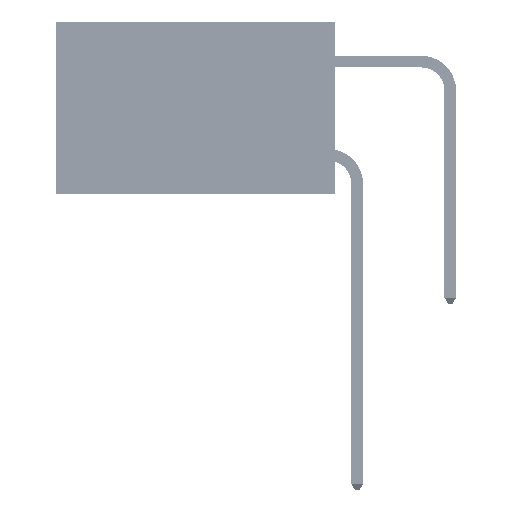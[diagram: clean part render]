
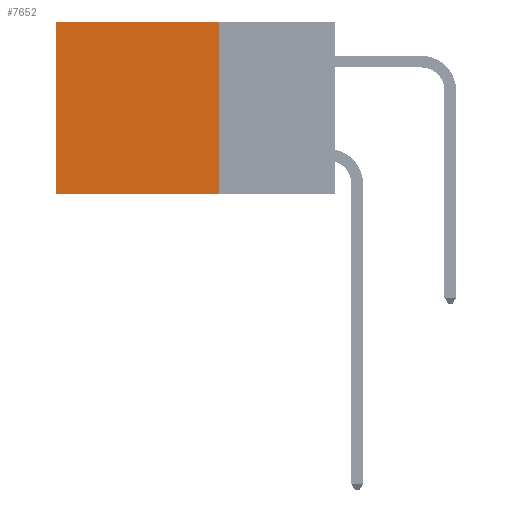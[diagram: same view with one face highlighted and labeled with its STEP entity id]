
A CAD part, left-side view. The second image highlights one B-rep face of the part: STEP entity #7652.
In plain terms, the highlighted planar face has unit normal (-1, 0, 0).
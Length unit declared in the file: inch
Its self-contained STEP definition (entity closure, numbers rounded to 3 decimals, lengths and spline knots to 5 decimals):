
#3206 = VECTOR ( 'NONE', #8260, 39.37008 ) ;
#3947 = CARTESIAN_POINT ( 'NONE',  ( 0.2875, 0.6, -0.37 ) ) ;
#4024 = ORIENTED_EDGE ( 'NONE', *, *, #30729, .T. ) ;
#4420 = DIRECTION ( 'NONE',  ( 1., 0., 0. ) ) ;
#4655 = LINE ( 'NONE', #29275, #22101 ) ;
#6683 = VERTEX_POINT ( 'NONE', #44051 ) ;
#7652 = ADVANCED_FACE ( 'NONE', ( #15387 ), #12106, .F. ) ;
#8260 = DIRECTION ( 'NONE',  ( 0., 0., -1. ) ) ;
#8763 = EDGE_CURVE ( 'NONE', #15794, #48832, #4655, .T. ) ;
#10193 = DIRECTION ( 'NONE',  ( 0., 0., -1. ) ) ;
#12106 = PLANE ( 'NONE',  #48205 ) ;
#13468 = DIRECTION ( 'NONE',  ( 0., 1., 0. ) ) ;
#15387 = FACE_OUTER_BOUND ( 'NONE', #47811, .T. ) ;
#15794 = VERTEX_POINT ( 'NONE', #34383 ) ;
#16084 = ORIENTED_EDGE ( 'NONE', *, *, #8763, .F. ) ;
#16486 = VERTEX_POINT ( 'NONE', #46278 ) ;
#20910 = VECTOR ( 'NONE', #50010, 39.37008 ) ;
#21160 = EDGE_CURVE ( 'NONE', #6683, #15794, #36263, .T. ) ;
#21309 = LINE ( 'NONE', #32335, #3206 ) ;
#22101 = VECTOR ( 'NONE', #13468, 39.37008 ) ;
#24994 = VECTOR ( 'NONE', #10193, 39.37008 ) ;
#25288 = LINE ( 'NONE', #25569, #20910 ) ;
#25569 = CARTESIAN_POINT ( 'NONE',  ( 0.2875, 0.25, 0. ) ) ;
#28267 = CARTESIAN_POINT ( 'NONE',  ( 0.2875, 0.25, 0. ) ) ;
#29275 = CARTESIAN_POINT ( 'NONE',  ( 0.2875, 0.25, -0.37 ) ) ;
#30729 = EDGE_CURVE ( 'NONE', #16486, #48832, #21309, .T. ) ;
#32173 = ORIENTED_EDGE ( 'NONE', *, *, #21160, .F. ) ;
#32323 = DIRECTION ( 'NONE',  ( 0., 0., -1. ) ) ;
#32335 = CARTESIAN_POINT ( 'NONE',  ( 0.2875, 0.6, 0. ) ) ;
#34071 = CARTESIAN_POINT ( 'NONE',  ( 0.2875, 0.25, 0. ) ) ;
#34383 = CARTESIAN_POINT ( 'NONE',  ( 0.2875, 0.25, -0.37 ) ) ;
#36263 = LINE ( 'NONE', #34071, #24994 ) ;
#38909 = ORIENTED_EDGE ( 'NONE', *, *, #47834, .T. ) ;
#44051 = CARTESIAN_POINT ( 'NONE',  ( 0.2875, 0.25, 0. ) ) ;
#46278 = CARTESIAN_POINT ( 'NONE',  ( 0.2875, 0.6, 0. ) ) ;
#47811 = EDGE_LOOP ( 'NONE', ( #4024, #16084, #32173, #38909 ) ) ;
#47834 = EDGE_CURVE ( 'NONE', #6683, #16486, #25288, .T. ) ;
#48205 = AXIS2_PLACEMENT_3D ( 'NONE', #28267, #4420, #32323 ) ;
#48832 = VERTEX_POINT ( 'NONE', #3947 ) ;
#50010 = DIRECTION ( 'NONE',  ( 0., 1., 0. ) ) ;
